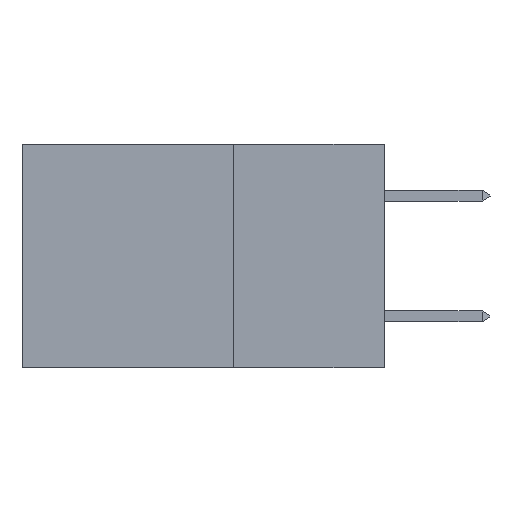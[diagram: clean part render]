
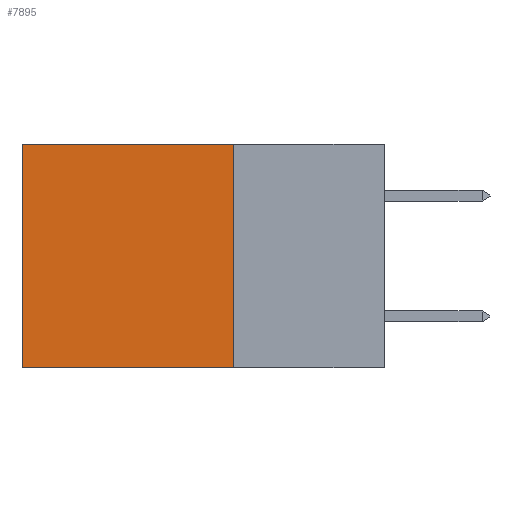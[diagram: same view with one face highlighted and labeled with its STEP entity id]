
A CAD part, left-side view. The second image highlights one B-rep face of the part: STEP entity #7895.
In plain terms, the highlighted planar face has unit normal (-1, 0, 0).
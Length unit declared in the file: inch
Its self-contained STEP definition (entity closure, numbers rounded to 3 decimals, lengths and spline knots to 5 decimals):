
#1433 = EDGE_CURVE ( 'NONE', #7456, #4642, #12026, .T. ) ;
#1624 = VECTOR ( 'NONE', #4698, 39.37008 ) ;
#1820 = DIRECTION ( 'NONE',  ( 0., 0., -1. ) ) ;
#1845 = CARTESIAN_POINT ( 'NONE',  ( 0.2875, 0.25, -0.37 ) ) ;
#1962 = CARTESIAN_POINT ( 'NONE',  ( 0.2875, 0.25, 0. ) ) ;
#2360 = CARTESIAN_POINT ( 'NONE',  ( 0.2875, 0.6, -0.37 ) ) ;
#2930 = PLANE ( 'NONE',  #5121 ) ;
#3366 = VERTEX_POINT ( 'NONE', #5030 ) ;
#3370 = ORIENTED_EDGE ( 'NONE', *, *, #10018, .F. ) ;
#3664 = VECTOR ( 'NONE', #5747, 39.37008 ) ;
#4427 = CARTESIAN_POINT ( 'NONE',  ( 0.2875, 0.6, 0. ) ) ;
#4642 = VERTEX_POINT ( 'NONE', #2360 ) ;
#4660 = DIRECTION ( 'NONE',  ( 0., 1., 0. ) ) ;
#4698 = DIRECTION ( 'NONE',  ( 0., 0., -1. ) ) ;
#5030 = CARTESIAN_POINT ( 'NONE',  ( 0.2875, 0.25, 0. ) ) ;
#5121 = AXIS2_PLACEMENT_3D ( 'NONE', #1962, #12204, #1820 ) ;
#5483 = VECTOR ( 'NONE', #4660, 39.37008 ) ;
#5613 = LINE ( 'NONE', #13542, #12703 ) ;
#5747 = DIRECTION ( 'NONE',  ( 0., 1., 0. ) ) ;
#6526 = EDGE_CURVE ( 'NONE', #3366, #13867, #13474, .T. ) ;
#6758 = ORIENTED_EDGE ( 'NONE', *, *, #1433, .F. ) ;
#7456 = VERTEX_POINT ( 'NONE', #11939 ) ;
#7539 = FACE_OUTER_BOUND ( 'NONE', #7665, .T. ) ;
#7658 = EDGE_CURVE ( 'NONE', #13867, #4642, #5613, .T. ) ;
#7665 = EDGE_LOOP ( 'NONE', ( #9604, #6758, #3370, #8361 ) ) ;
#7895 = ADVANCED_FACE ( 'NONE', ( #7539 ), #2930, .F. ) ;
#8047 = DIRECTION ( 'NONE',  ( 0., 0., -1. ) ) ;
#8361 = ORIENTED_EDGE ( 'NONE', *, *, #6526, .T. ) ;
#9604 = ORIENTED_EDGE ( 'NONE', *, *, #7658, .T. ) ;
#10018 = EDGE_CURVE ( 'NONE', #3366, #7456, #13962, .T. ) ;
#11939 = CARTESIAN_POINT ( 'NONE',  ( 0.2875, 0.25, -0.37 ) ) ;
#12026 = LINE ( 'NONE', #1845, #5483 ) ;
#12204 = DIRECTION ( 'NONE',  ( 1., 0., 0. ) ) ;
#12430 = CARTESIAN_POINT ( 'NONE',  ( 0.2875, 0.25, 0. ) ) ;
#12703 = VECTOR ( 'NONE', #8047, 39.37008 ) ;
#12843 = CARTESIAN_POINT ( 'NONE',  ( 0.2875, 0.25, 0. ) ) ;
#13474 = LINE ( 'NONE', #12430, #3664 ) ;
#13542 = CARTESIAN_POINT ( 'NONE',  ( 0.2875, 0.6, 0. ) ) ;
#13867 = VERTEX_POINT ( 'NONE', #4427 ) ;
#13962 = LINE ( 'NONE', #12843, #1624 ) ;
